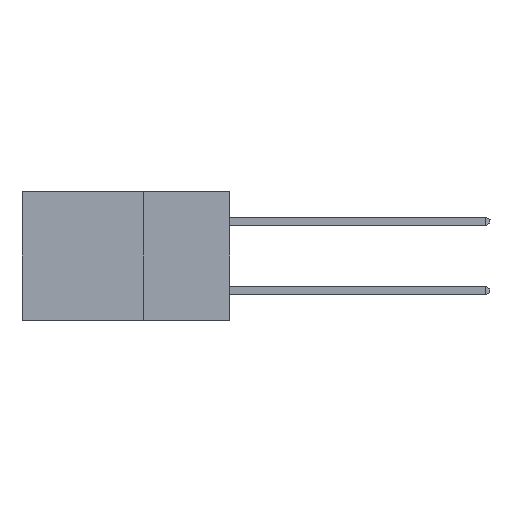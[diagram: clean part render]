
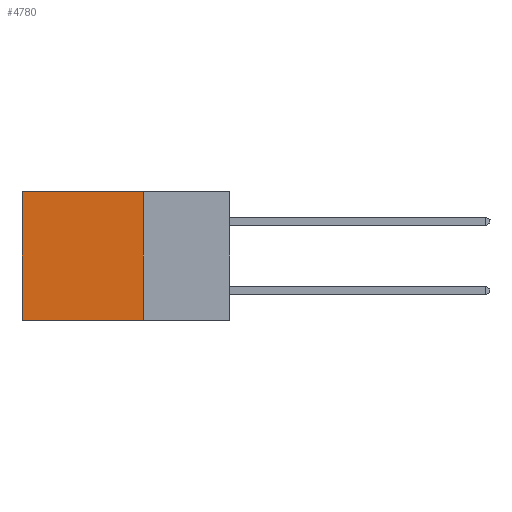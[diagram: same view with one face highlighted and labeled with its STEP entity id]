
A CAD part, left-side view. The second image highlights one B-rep face of the part: STEP entity #4780.
In plain terms, the highlighted planar face has unit normal (-1, 0, 0).
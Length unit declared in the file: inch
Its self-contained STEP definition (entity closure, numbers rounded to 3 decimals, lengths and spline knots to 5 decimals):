
#165 = VERTEX_POINT ( 'NONE', #8603 ) ;
#167 = VECTOR ( 'NONE', #11630, 39.37008 ) ;
#2779 = CARTESIAN_POINT ( 'NONE',  ( 0.298, 0.25, -0.37 ) ) ;
#3098 = DIRECTION ( 'NONE',  ( 0., 0., -1. ) ) ;
#3632 = EDGE_CURVE ( 'NONE', #165, #21751, #26230, .T. ) ;
#4780 = ADVANCED_FACE ( 'NONE', ( #18225 ), #24703, .F. ) ;
#5083 = EDGE_LOOP ( 'NONE', ( #18519, #8537, #28317, #11917 ) ) ;
#7320 = EDGE_CURVE ( 'NONE', #15206, #165, #28105, .T. ) ;
#7375 = CARTESIAN_POINT ( 'NONE',  ( 0.298, 0.6, 0. ) ) ;
#7938 = VECTOR ( 'NONE', #13740, 39.37008 ) ;
#8094 = CARTESIAN_POINT ( 'NONE',  ( 0.298, 0.25, 0. ) ) ;
#8537 = ORIENTED_EDGE ( 'NONE', *, *, #16070, .F. ) ;
#8603 = CARTESIAN_POINT ( 'NONE',  ( 0.298, 0.6, 0. ) ) ;
#11630 = DIRECTION ( 'NONE',  ( 0., 1., 0. ) ) ;
#11917 = ORIENTED_EDGE ( 'NONE', *, *, #7320, .T. ) ;
#13740 = DIRECTION ( 'NONE',  ( 0., 0., -1. ) ) ;
#14674 = CARTESIAN_POINT ( 'NONE',  ( 0.298, 0.25, 0. ) ) ;
#14757 = VERTEX_POINT ( 'NONE', #21949 ) ;
#15206 = VERTEX_POINT ( 'NONE', #8094 ) ;
#15642 = CARTESIAN_POINT ( 'NONE',  ( 0.298, 0.25, 0. ) ) ;
#16070 = EDGE_CURVE ( 'NONE', #14757, #21751, #28529, .T. ) ;
#16897 = DIRECTION ( 'NONE',  ( 0., 1., 0. ) ) ;
#17885 = DIRECTION ( 'NONE',  ( 1., 0., 0. ) ) ;
#18225 = FACE_OUTER_BOUND ( 'NONE', #5083, .T. ) ;
#18519 = ORIENTED_EDGE ( 'NONE', *, *, #3632, .T. ) ;
#19479 = AXIS2_PLACEMENT_3D ( 'NONE', #15642, #17885, #3098 ) ;
#21751 = VERTEX_POINT ( 'NONE', #24180 ) ;
#21949 = CARTESIAN_POINT ( 'NONE',  ( 0.298, 0.25, -0.37 ) ) ;
#23278 = VECTOR ( 'NONE', #16897, 39.37008 ) ;
#23404 = LINE ( 'NONE', #28277, #24765 ) ;
#24180 = CARTESIAN_POINT ( 'NONE',  ( 0.298, 0.6, -0.37 ) ) ;
#24703 = PLANE ( 'NONE',  #19479 ) ;
#24765 = VECTOR ( 'NONE', #26429, 39.37008 ) ;
#26230 = LINE ( 'NONE', #7375, #7938 ) ;
#26429 = DIRECTION ( 'NONE',  ( 0., 0., -1. ) ) ;
#28105 = LINE ( 'NONE', #14674, #23278 ) ;
#28108 = EDGE_CURVE ( 'NONE', #15206, #14757, #23404, .T. ) ;
#28277 = CARTESIAN_POINT ( 'NONE',  ( 0.298, 0.25, 0. ) ) ;
#28317 = ORIENTED_EDGE ( 'NONE', *, *, #28108, .F. ) ;
#28529 = LINE ( 'NONE', #2779, #167 ) ;
